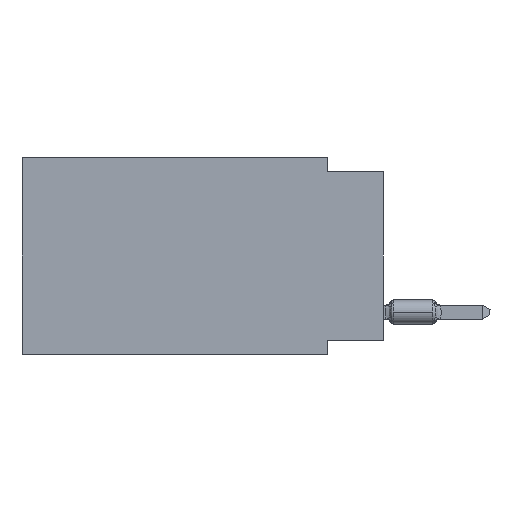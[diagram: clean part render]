
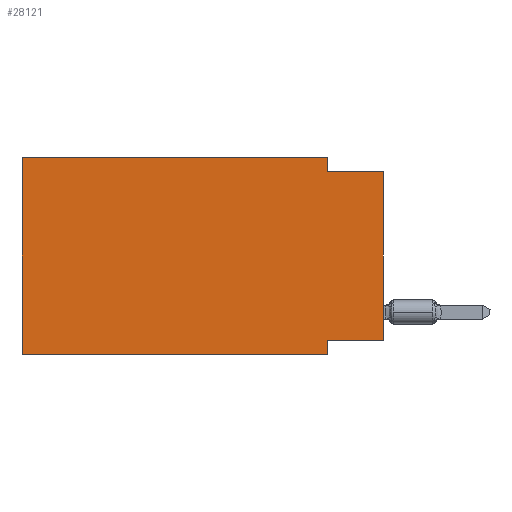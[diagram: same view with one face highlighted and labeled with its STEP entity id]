
A CAD part, left-side view. The second image highlights one B-rep face of the part: STEP entity #28121.
In plain terms, the highlighted planar face has unit normal (-1, 0, 0).
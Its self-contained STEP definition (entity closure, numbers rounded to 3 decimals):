
#1190 = LINE ( 'NONE', #48621, #43944 ) ;
#1879 = VERTEX_POINT ( 'NONE', #10288 ) ;
#1887 = ORIENTED_EDGE ( 'NONE', *, *, #24740, .F. ) ;
#1904 = VECTOR ( 'NONE', #41619, 1000. ) ;
#2368 = EDGE_CURVE ( 'NONE', #59795, #6233, #1190, .T. ) ;
#3213 = VECTOR ( 'NONE', #16818, 1000. ) ;
#4301 = ORIENTED_EDGE ( 'NONE', *, *, #20463, .F. ) ;
#4959 = FACE_OUTER_BOUND ( 'NONE', #47881, .T. ) ;
#6233 = VERTEX_POINT ( 'NONE', #32923 ) ;
#9218 = VECTOR ( 'NONE', #17511, 1000. ) ;
#9381 = LINE ( 'NONE', #33854, #53088 ) ;
#10024 = CARTESIAN_POINT ( 'NONE',  ( 0., 2.54, -8.89 ) ) ;
#10147 = CARTESIAN_POINT ( 'NONE',  ( 0., 0., -8.255 ) ) ;
#10288 = CARTESIAN_POINT ( 'NONE',  ( 0., 0., -0.635 ) ) ;
#12778 = ORIENTED_EDGE ( 'NONE', *, *, #51772, .T. ) ;
#12807 = LINE ( 'NONE', #43229, #39006 ) ;
#14208 = PLANE ( 'NONE',  #29032 ) ;
#15503 = EDGE_CURVE ( 'NONE', #42086, #59795, #9381, .T. ) ;
#16792 = ORIENTED_EDGE ( 'NONE', *, *, #38628, .F. ) ;
#16818 = DIRECTION ( 'NONE',  ( 0., -1., 0. ) ) ;
#17511 = DIRECTION ( 'NONE',  ( 0., 0., -1. ) ) ;
#17568 = DIRECTION ( 'NONE',  ( 0., 0., 1. ) ) ;
#18700 = LINE ( 'NONE', #59351, #32100 ) ;
#19927 = DIRECTION ( 'NONE',  ( 1., 0., 0. ) ) ;
#20463 = EDGE_CURVE ( 'NONE', #62746, #50711, #50601, .T. ) ;
#23896 = LINE ( 'NONE', #61164, #57548 ) ;
#24135 = ORIENTED_EDGE ( 'NONE', *, *, #35541, .T. ) ;
#24740 = EDGE_CURVE ( 'NONE', #24817, #62746, #12807, .T. ) ;
#24817 = VERTEX_POINT ( 'NONE', #10147 ) ;
#28121 = ADVANCED_FACE ( 'NONE', ( #4959 ), #14208, .F. ) ;
#29032 = AXIS2_PLACEMENT_3D ( 'NONE', #38050, #19927, #44089 ) ;
#30834 = LINE ( 'NONE', #40689, #1904 ) ;
#32100 = VECTOR ( 'NONE', #35140, 1000. ) ;
#32923 = CARTESIAN_POINT ( 'NONE',  ( 0., 2.54, 0. ) ) ;
#33854 = CARTESIAN_POINT ( 'NONE',  ( 0., 16.383, 0. ) ) ;
#35140 = DIRECTION ( 'NONE',  ( 0., -1., 0. ) ) ;
#35541 = EDGE_CURVE ( 'NONE', #24817, #1879, #23896, .T. ) ;
#36457 = CARTESIAN_POINT ( 'NONE',  ( 0., 16.383, 0. ) ) ;
#36511 = CARTESIAN_POINT ( 'NONE',  ( 0., 0., -0.635 ) ) ;
#38050 = CARTESIAN_POINT ( 'NONE',  ( 0., 16.383, 0. ) ) ;
#38628 = EDGE_CURVE ( 'NONE', #6233, #47931, #30834, .T. ) ;
#38946 = DIRECTION ( 'NONE',  ( 0., 0., 1. ) ) ;
#39006 = VECTOR ( 'NONE', #46839, 1000. ) ;
#40689 = CARTESIAN_POINT ( 'NONE',  ( 0., 2.54, 0. ) ) ;
#41619 = DIRECTION ( 'NONE',  ( 0., 0., -1. ) ) ;
#42086 = VERTEX_POINT ( 'NONE', #48490 ) ;
#43229 = CARTESIAN_POINT ( 'NONE',  ( 0., 0., -8.255 ) ) ;
#43944 = VECTOR ( 'NONE', #54045, 1000. ) ;
#44089 = DIRECTION ( 'NONE',  ( 0., 0., -1. ) ) ;
#44421 = CARTESIAN_POINT ( 'NONE',  ( 0., 2.54, -0.635 ) ) ;
#46142 = CARTESIAN_POINT ( 'NONE',  ( 0., 2.54, -8.89 ) ) ;
#46839 = DIRECTION ( 'NONE',  ( 0., 1., 0. ) ) ;
#47881 = EDGE_LOOP ( 'NONE', ( #24135, #61440, #16792, #54745, #59787, #12778, #4301, #1887 ) ) ;
#47931 = VERTEX_POINT ( 'NONE', #44421 ) ;
#48490 = CARTESIAN_POINT ( 'NONE',  ( 0., 16.383, -8.89 ) ) ;
#48621 = CARTESIAN_POINT ( 'NONE',  ( 0., 16.383, 0. ) ) ;
#48915 = EDGE_CURVE ( 'NONE', #47931, #1879, #60414, .T. ) ;
#50316 = CARTESIAN_POINT ( 'NONE',  ( 0., 2.54, -8.255 ) ) ;
#50601 = LINE ( 'NONE', #46142, #9218 ) ;
#50711 = VERTEX_POINT ( 'NONE', #10024 ) ;
#51772 = EDGE_CURVE ( 'NONE', #42086, #50711, #18700, .T. ) ;
#53088 = VECTOR ( 'NONE', #38946, 1000. ) ;
#54045 = DIRECTION ( 'NONE',  ( 0., -1., 0. ) ) ;
#54745 = ORIENTED_EDGE ( 'NONE', *, *, #2368, .F. ) ;
#57548 = VECTOR ( 'NONE', #17568, 1000. ) ;
#59351 = CARTESIAN_POINT ( 'NONE',  ( 0., 16.383, -8.89 ) ) ;
#59787 = ORIENTED_EDGE ( 'NONE', *, *, #15503, .F. ) ;
#59795 = VERTEX_POINT ( 'NONE', #36457 ) ;
#60414 = LINE ( 'NONE', #36511, #3213 ) ;
#61164 = CARTESIAN_POINT ( 'NONE',  ( 0., 0., 0. ) ) ;
#61440 = ORIENTED_EDGE ( 'NONE', *, *, #48915, .F. ) ;
#62746 = VERTEX_POINT ( 'NONE', #50316 ) ;
